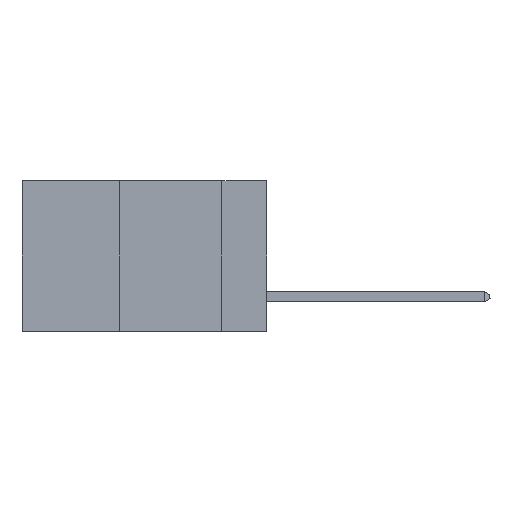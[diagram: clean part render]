
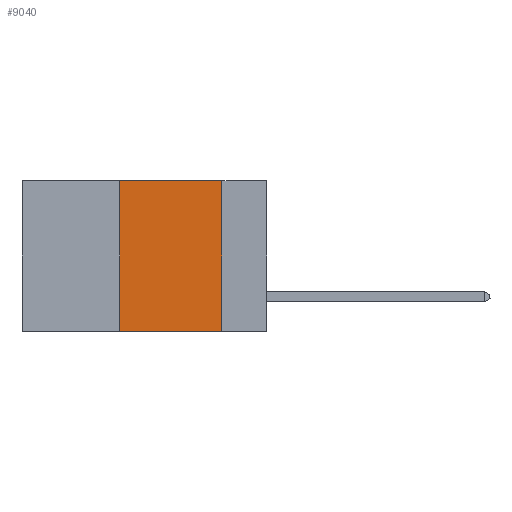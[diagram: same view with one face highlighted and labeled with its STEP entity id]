
A CAD part, left-side view. The second image highlights one B-rep face of the part: STEP entity #9040.
In plain terms, the highlighted planar face has unit normal (-1, 0, 0).
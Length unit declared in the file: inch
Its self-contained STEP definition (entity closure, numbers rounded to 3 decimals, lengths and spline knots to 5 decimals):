
#1007 = VECTOR ( 'NONE', #17786, 39.37008 ) ;
#1071 = EDGE_LOOP ( 'NONE', ( #9867, #25216, #20232, #26372 ) ) ;
#1509 = DIRECTION ( 'NONE',  ( 0., -1., 0. ) ) ;
#1828 = DIRECTION ( 'NONE',  ( 0., 0., -1. ) ) ;
#2062 = CARTESIAN_POINT ( 'NONE',  ( 0., 0.36, 0. ) ) ;
#4270 = VERTEX_POINT ( 'NONE', #24336 ) ;
#4368 = DIRECTION ( 'NONE',  ( 1., 0., 0. ) ) ;
#5097 = VECTOR ( 'NONE', #1509, 39.37008 ) ;
#6299 = VERTEX_POINT ( 'NONE', #2062 ) ;
#7019 = VERTEX_POINT ( 'NONE', #16713 ) ;
#7475 = CARTESIAN_POINT ( 'NONE',  ( 0., 0.6, 0. ) ) ;
#9040 = ADVANCED_FACE ( 'NONE', ( #17978 ), #32326, .F. ) ;
#9867 = ORIENTED_EDGE ( 'NONE', *, *, #23518, .F. ) ;
#11842 = LINE ( 'NONE', #7475, #24995 ) ;
#13866 = EDGE_CURVE ( 'NONE', #22563, #4270, #17886, .T. ) ;
#16713 = CARTESIAN_POINT ( 'NONE',  ( 0., 0.11, 0. ) ) ;
#17086 = CARTESIAN_POINT ( 'NONE',  ( 0., 0.6, 0. ) ) ;
#17786 = DIRECTION ( 'NONE',  ( 0., 0., 1. ) ) ;
#17886 = LINE ( 'NONE', #26753, #5097 ) ;
#17978 = FACE_OUTER_BOUND ( 'NONE', #1071, .T. ) ;
#19874 = DIRECTION ( 'NONE',  ( 0., -1., 0. ) ) ;
#20232 = ORIENTED_EDGE ( 'NONE', *, *, #29372, .F. ) ;
#22563 = VERTEX_POINT ( 'NONE', #31749 ) ;
#23518 = EDGE_CURVE ( 'NONE', #7019, #4270, #25077, .T. ) ;
#24336 = CARTESIAN_POINT ( 'NONE',  ( 0., 0.11, -0.37 ) ) ;
#24995 = VECTOR ( 'NONE', #19874, 39.37008 ) ;
#25077 = LINE ( 'NONE', #27637, #26297 ) ;
#25178 = DIRECTION ( 'NONE',  ( 0., 0., -1. ) ) ;
#25216 = ORIENTED_EDGE ( 'NONE', *, *, #31067, .F. ) ;
#26297 = VECTOR ( 'NONE', #25178, 39.37008 ) ;
#26372 = ORIENTED_EDGE ( 'NONE', *, *, #13866, .T. ) ;
#26753 = CARTESIAN_POINT ( 'NONE',  ( 0., 0.6, -0.37 ) ) ;
#27637 = CARTESIAN_POINT ( 'NONE',  ( 0., 0.11, 0. ) ) ;
#28452 = LINE ( 'NONE', #30445, #1007 ) ;
#28751 = AXIS2_PLACEMENT_3D ( 'NONE', #17086, #4368, #1828 ) ;
#29372 = EDGE_CURVE ( 'NONE', #22563, #6299, #28452, .T. ) ;
#30445 = CARTESIAN_POINT ( 'NONE',  ( 0., 0.36, 0. ) ) ;
#31067 = EDGE_CURVE ( 'NONE', #6299, #7019, #11842, .T. ) ;
#31749 = CARTESIAN_POINT ( 'NONE',  ( 0., 0.36, -0.37 ) ) ;
#32326 = PLANE ( 'NONE',  #28751 ) ;
